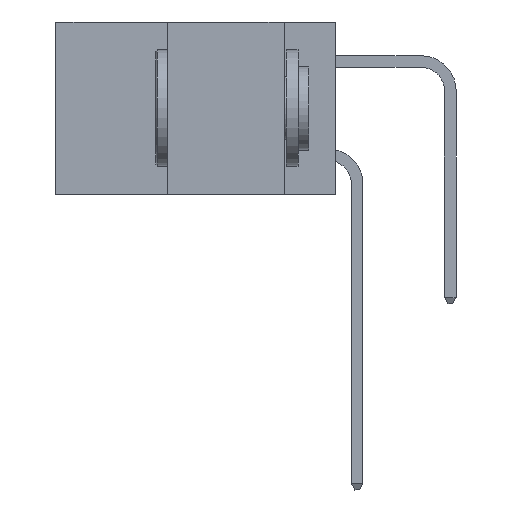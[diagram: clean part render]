
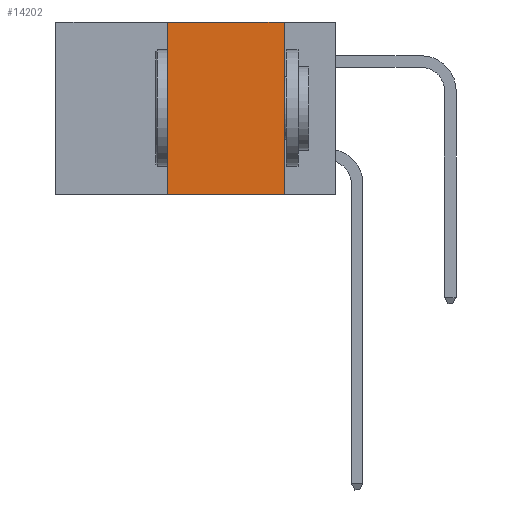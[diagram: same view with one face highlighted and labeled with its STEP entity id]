
A CAD part, left-side view. The second image highlights one B-rep face of the part: STEP entity #14202.
In plain terms, the highlighted planar face has unit normal (-1, 0, 0).
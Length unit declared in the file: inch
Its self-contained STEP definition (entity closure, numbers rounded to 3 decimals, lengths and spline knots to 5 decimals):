
#308 = EDGE_CURVE ( 'NONE', #7679, #15480, #2812, .T. ) ;
#353 = EDGE_CURVE ( 'NONE', #2310, #3672, #16805, .T. ) ;
#358 = EDGE_CURVE ( 'NONE', #2310, #15480, #16207, .T. ) ;
#1002 = VECTOR ( 'NONE', #11876, 39.37008 ) ;
#1572 = VECTOR ( 'NONE', #14671, 39.37008 ) ;
#2114 = CARTESIAN_POINT ( 'NONE',  ( 0., 0.36, 0. ) ) ;
#2310 = VERTEX_POINT ( 'NONE', #8073 ) ;
#2674 = DIRECTION ( 'NONE',  ( 1., 0., 0. ) ) ;
#2812 = LINE ( 'NONE', #24159, #17400 ) ;
#3672 = VERTEX_POINT ( 'NONE', #21379 ) ;
#4778 = DIRECTION ( 'NONE',  ( 0., -1., 0. ) ) ;
#5022 = CARTESIAN_POINT ( 'NONE',  ( 0., 0.11, -0.37 ) ) ;
#6443 = PLANE ( 'NONE',  #6479 ) ;
#6479 = AXIS2_PLACEMENT_3D ( 'NONE', #14123, #2674, #15993 ) ;
#7679 = VERTEX_POINT ( 'NONE', #21163 ) ;
#8073 = CARTESIAN_POINT ( 'NONE',  ( 0., 0.36, -0.37 ) ) ;
#10459 = CARTESIAN_POINT ( 'NONE',  ( 0., 0.6, 0. ) ) ;
#11129 = CARTESIAN_POINT ( 'NONE',  ( 0., 0.6, -0.37 ) ) ;
#11244 = EDGE_LOOP ( 'NONE', ( #22712, #13910, #14954, #22009 ) ) ;
#11876 = DIRECTION ( 'NONE',  ( 0., -1., 0. ) ) ;
#11909 = VECTOR ( 'NONE', #4778, 39.37008 ) ;
#12503 = LINE ( 'NONE', #10459, #11909 ) ;
#13910 = ORIENTED_EDGE ( 'NONE', *, *, #22468, .F. ) ;
#14123 = CARTESIAN_POINT ( 'NONE',  ( 0., 0.6, 0. ) ) ;
#14202 = ADVANCED_FACE ( 'NONE', ( #22894 ), #6443, .F. ) ;
#14671 = DIRECTION ( 'NONE',  ( 0., 0., 1. ) ) ;
#14954 = ORIENTED_EDGE ( 'NONE', *, *, #353, .F. ) ;
#15480 = VERTEX_POINT ( 'NONE', #5022 ) ;
#15993 = DIRECTION ( 'NONE',  ( 0., 0., -1. ) ) ;
#16207 = LINE ( 'NONE', #11129, #1002 ) ;
#16805 = LINE ( 'NONE', #2114, #1572 ) ;
#17400 = VECTOR ( 'NONE', #23685, 39.37008 ) ;
#21163 = CARTESIAN_POINT ( 'NONE',  ( 0., 0.11, 0. ) ) ;
#21379 = CARTESIAN_POINT ( 'NONE',  ( 0., 0.36, 0. ) ) ;
#22009 = ORIENTED_EDGE ( 'NONE', *, *, #358, .T. ) ;
#22468 = EDGE_CURVE ( 'NONE', #3672, #7679, #12503, .T. ) ;
#22712 = ORIENTED_EDGE ( 'NONE', *, *, #308, .F. ) ;
#22894 = FACE_OUTER_BOUND ( 'NONE', #11244, .T. ) ;
#23685 = DIRECTION ( 'NONE',  ( 0., 0., -1. ) ) ;
#24159 = CARTESIAN_POINT ( 'NONE',  ( 0., 0.11, 0. ) ) ;
